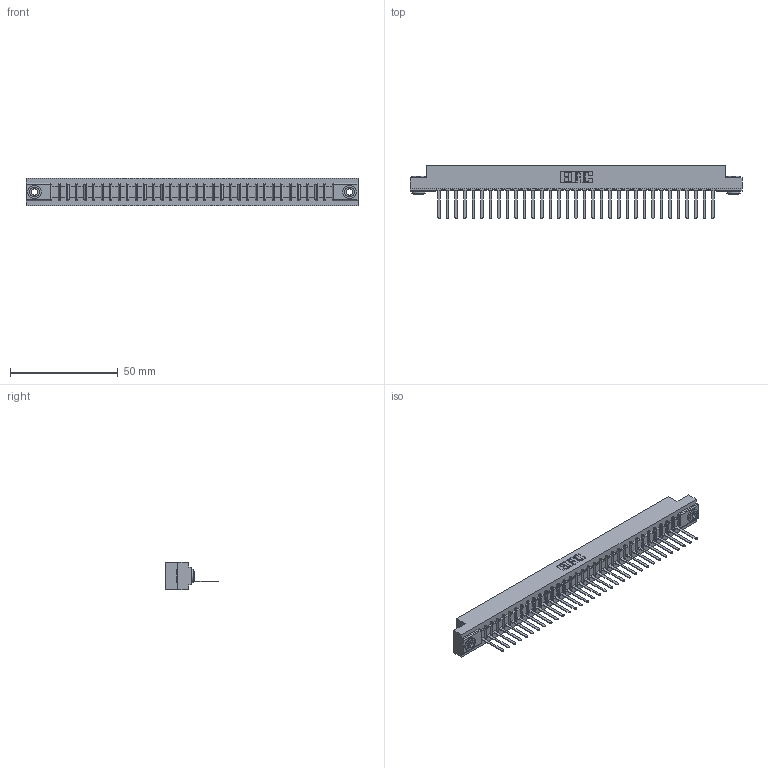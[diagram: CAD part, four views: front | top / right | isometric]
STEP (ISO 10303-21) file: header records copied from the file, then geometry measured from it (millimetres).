
FILE_DESCRIPTION (( 'STEP AP203' ), '1' );
FILE_NAME ('307-033-541-103.STEP', '2018-08-04T23:55:28', ( '' ), ( '' ), 'SwSTEP 2.0', 'SolidWorks 2016', '' );
FILE_SCHEMA (( 'CONFIG_CONTROL_DESIGN' ));
Length unit declared in the file: inch
Products named in the file (4): 345-250-002_345-250-002-102; 307-033-541-103; 307 Part_.156 Dia Mounting Holes; 307-290-002_541
Assembly tree (36 placements, depth 2):
  307-033-541-103
    307 Part_.156 Dia Mounting Holes
    307-290-002_541  x33
    345-250-002_345-250-002-102  x2
Bounding box: 153.77 x 24.59 x 12.7 mm (x, y, z)
Volume: 16482.8 mm3; surface area: 21376.3 mm2
Topology: 36 solids, 36 shells, 2646 faces, 8091 edges, 5298 vertices
Faces by surface type: plane 1579, cylinder 991, sphere 68, cone 8
Entity records: 31183 total; most frequent: CARTESIAN_POINT 5237, ORIENTED_EDGE 5218, DIRECTION 5107, EDGE_CURVE 2609, VECTOR 1987, LINE 1987, VERTEX_POINT 1690, AXIS2_PLACEMENT_3D 1560
